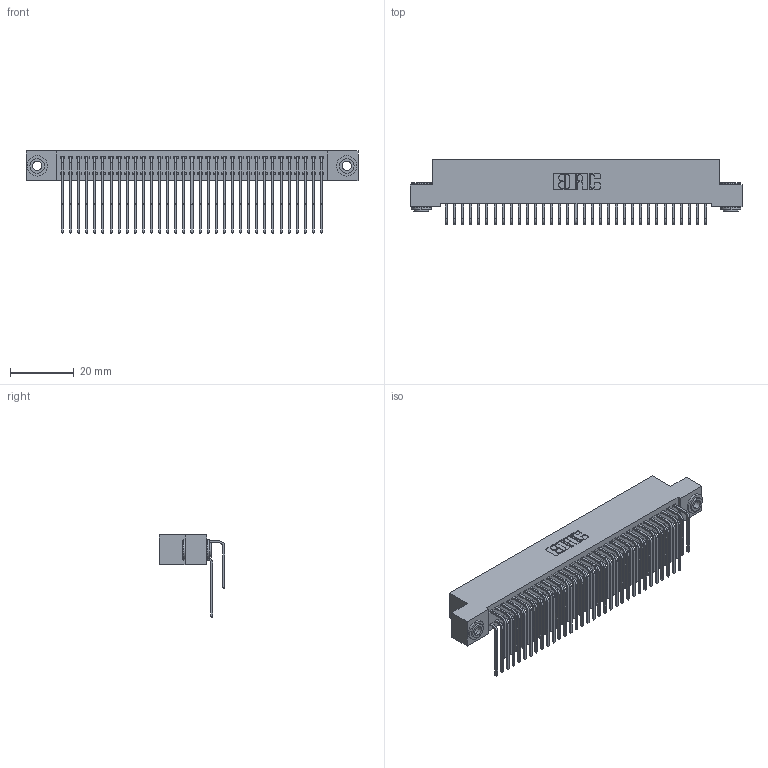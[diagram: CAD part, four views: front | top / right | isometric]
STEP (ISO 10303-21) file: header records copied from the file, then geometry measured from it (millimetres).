
FILE_DESCRIPTION (( 'STEP AP203' ), '1' );
FILE_NAME ('392-066-559-203.STEP', '2019-10-09T11:25:21', ( '' ), ( '' ), 'SwSTEP 2.0', 'SolidWorks 2016', '' );
FILE_SCHEMA (( 'CONFIG_CONTROL_DESIGN' ));
Length unit declared in the file: inch
Products named in the file (5): 342 Part_.156 TH; 345-292-001_558 559 Tail - 1; 345-292-001_559 Tail - 2; 342-250-002_345-250-002-102; 392-066-559-203
Assembly tree (69 placements, depth 2):
  392-066-559-203
    342 Part_.156 TH
    345-292-001_558 559 Tail - 1  x33
    345-292-001_559 Tail - 2  x33
    342-250-002_345-250-002-102  x2
Bounding box: 104.14 x 20.64 x 25.78 mm (x, y, z)
Volume: 9717.9 mm3; surface area: 17533 mm2
Topology: 69 solids, 69 shells, 3712 faces, 11001 edges, 7242 vertices
Faces by surface type: plane 2584, cylinder 1120, cone 8
Entity records: 24696 total; most frequent: CARTESIAN_POINT 4128, ORIENTED_EDGE 4006, DIRECTION 3557, EDGE_CURVE 2003, LINE 1811, VECTOR 1811, VERTEX_POINT 1330, AXIS2_PLACEMENT_3D 873
